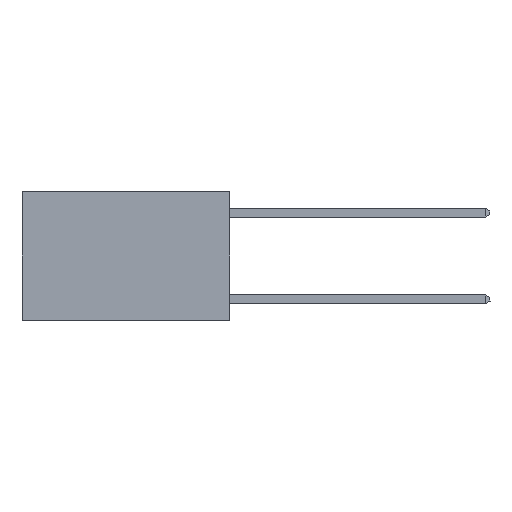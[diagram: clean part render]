
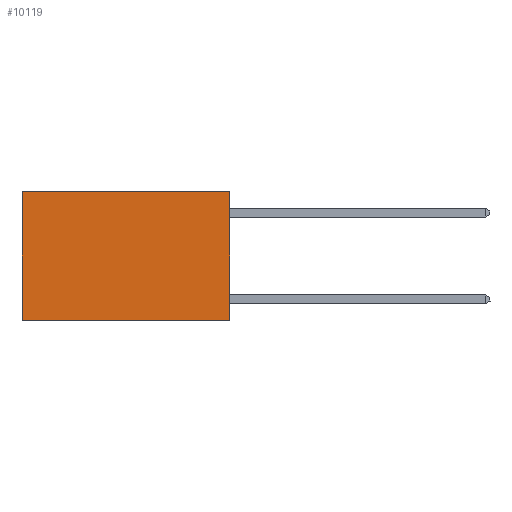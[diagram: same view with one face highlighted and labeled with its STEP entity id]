
A CAD part, left-side view. The second image highlights one B-rep face of the part: STEP entity #10119.
In plain terms, the highlighted planar face has unit normal (-1, 0, 0).
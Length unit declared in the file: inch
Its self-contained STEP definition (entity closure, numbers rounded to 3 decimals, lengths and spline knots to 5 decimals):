
#171 = EDGE_CURVE ( 'NONE', #15376, #18741, #2163, .T. ) ;
#189 = DIRECTION ( 'NONE',  ( 1., 0., 0. ) ) ;
#791 = CARTESIAN_POINT ( 'NONE',  ( 0.2625, 0., -0.37 ) ) ;
#1421 = LINE ( 'NONE', #14480, #5842 ) ;
#1458 = CARTESIAN_POINT ( 'NONE',  ( 0.2625, 0.6, -0.37 ) ) ;
#1977 = CARTESIAN_POINT ( 'NONE',  ( 0.2625, 0., 0. ) ) ;
#2152 = CARTESIAN_POINT ( 'NONE',  ( 0.2625, 0., -0.37 ) ) ;
#2163 = LINE ( 'NONE', #791, #9543 ) ;
#2506 = LINE ( 'NONE', #10312, #9889 ) ;
#2984 = ORIENTED_EDGE ( 'NONE', *, *, #171, .F. ) ;
#3472 = CARTESIAN_POINT ( 'NONE',  ( 0.2625, 0., 0. ) ) ;
#4283 = DIRECTION ( 'NONE',  ( 0., 0., -1. ) ) ;
#4455 = DIRECTION ( 'NONE',  ( 0., 0., -1. ) ) ;
#5842 = VECTOR ( 'NONE', #4283, 39.37008 ) ;
#9021 = ORIENTED_EDGE ( 'NONE', *, *, #13856, .T. ) ;
#9543 = VECTOR ( 'NONE', #11345, 39.37008 ) ;
#9889 = VECTOR ( 'NONE', #4455, 39.37008 ) ;
#10119 = ADVANCED_FACE ( 'NONE', ( #11348 ), #13678, .F. ) ;
#10312 = CARTESIAN_POINT ( 'NONE',  ( 0.2625, 0.6, 0. ) ) ;
#10477 = DIRECTION ( 'NONE',  ( 0., 0., -1. ) ) ;
#10868 = VERTEX_POINT ( 'NONE', #14926 ) ;
#11345 = DIRECTION ( 'NONE',  ( 0., 1., 0. ) ) ;
#11348 = FACE_OUTER_BOUND ( 'NONE', #15370, .T. ) ;
#11487 = VECTOR ( 'NONE', #16594, 39.37008 ) ;
#12127 = EDGE_CURVE ( 'NONE', #10868, #17934, #15364, .T. ) ;
#12553 = AXIS2_PLACEMENT_3D ( 'NONE', #1977, #189, #10477 ) ;
#13678 = PLANE ( 'NONE',  #12553 ) ;
#13856 = EDGE_CURVE ( 'NONE', #17934, #18741, #2506, .T. ) ;
#14468 = CARTESIAN_POINT ( 'NONE',  ( 0.2625, 0.6, 0. ) ) ;
#14480 = CARTESIAN_POINT ( 'NONE',  ( 0.2625, 0., 0. ) ) ;
#14926 = CARTESIAN_POINT ( 'NONE',  ( 0.2625, 0., 0. ) ) ;
#15364 = LINE ( 'NONE', #3472, #11487 ) ;
#15370 = EDGE_LOOP ( 'NONE', ( #9021, #2984, #17502, #18792 ) ) ;
#15376 = VERTEX_POINT ( 'NONE', #2152 ) ;
#16594 = DIRECTION ( 'NONE',  ( 0., 1., 0. ) ) ;
#17409 = EDGE_CURVE ( 'NONE', #10868, #15376, #1421, .T. ) ;
#17502 = ORIENTED_EDGE ( 'NONE', *, *, #17409, .F. ) ;
#17934 = VERTEX_POINT ( 'NONE', #14468 ) ;
#18741 = VERTEX_POINT ( 'NONE', #1458 ) ;
#18792 = ORIENTED_EDGE ( 'NONE', *, *, #12127, .T. ) ;
